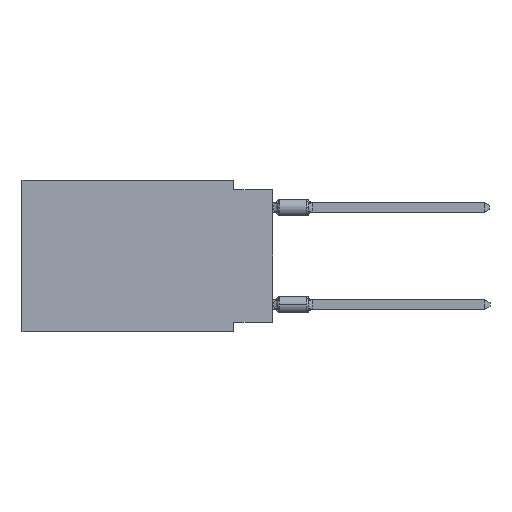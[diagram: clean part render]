
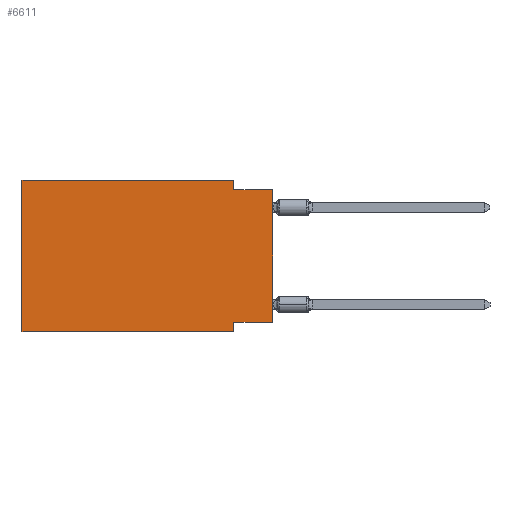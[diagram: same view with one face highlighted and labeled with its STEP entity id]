
A CAD part, left-side view. The second image highlights one B-rep face of the part: STEP entity #6611.
In plain terms, the highlighted planar face has unit normal (-1, 0, 0).
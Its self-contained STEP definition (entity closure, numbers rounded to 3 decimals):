
#212 = FACE_OUTER_BOUND ( 'NONE', #12489, .T. ) ;
#368 = LINE ( 'NONE', #21685, #13185 ) ;
#788 = VECTOR ( 'NONE', #5317, 1000. ) ;
#1435 = ORIENTED_EDGE ( 'NONE', *, *, #8250, .F. ) ;
#1480 = CARTESIAN_POINT ( 'NONE',  ( 0., 16.383, 0. ) ) ;
#1493 = CARTESIAN_POINT ( 'NONE',  ( 0., 0., -9.271 ) ) ;
#1527 = EDGE_CURVE ( 'NONE', #22306, #7343, #13561, .T. ) ;
#1873 = ORIENTED_EDGE ( 'NONE', *, *, #10326, .T. ) ;
#1948 = CARTESIAN_POINT ( 'NONE',  ( 0., 16.383, 0. ) ) ;
#1962 = CARTESIAN_POINT ( 'NONE',  ( 0., 2.54, -9.271 ) ) ;
#2350 = CARTESIAN_POINT ( 'NONE',  ( 0., 16.383, 0. ) ) ;
#2560 = DIRECTION ( 'NONE',  ( 0., 0., -1. ) ) ;
#2696 = CARTESIAN_POINT ( 'NONE',  ( 0., 16.383, -9.906 ) ) ;
#3153 = EDGE_CURVE ( 'NONE', #20212, #21137, #6985, .T. ) ;
#3161 = ORIENTED_EDGE ( 'NONE', *, *, #3596, .F. ) ;
#3207 = LINE ( 'NONE', #1480, #19437 ) ;
#3569 = VECTOR ( 'NONE', #8498, 1000. ) ;
#3596 = EDGE_CURVE ( 'NONE', #20198, #20212, #368, .T. ) ;
#3820 = EDGE_CURVE ( 'NONE', #22144, #9013, #8529, .T. ) ;
#4472 = AXIS2_PLACEMENT_3D ( 'NONE', #1948, #8731, #8949 ) ;
#5317 = DIRECTION ( 'NONE',  ( 0., 0., 1. ) ) ;
#6611 = ADVANCED_FACE ( 'NONE', ( #212 ), #10436, .F. ) ;
#6985 = LINE ( 'NONE', #20714, #8744 ) ;
#7090 = DIRECTION ( 'NONE',  ( 0., -1., 0. ) ) ;
#7343 = VERTEX_POINT ( 'NONE', #22414 ) ;
#8193 = DIRECTION ( 'NONE',  ( 0., -1., 0. ) ) ;
#8219 = ORIENTED_EDGE ( 'NONE', *, *, #3820, .F. ) ;
#8250 = EDGE_CURVE ( 'NONE', #9013, #20198, #3207, .T. ) ;
#8498 = DIRECTION ( 'NONE',  ( 0., 1., 0. ) ) ;
#8529 = LINE ( 'NONE', #10350, #10602 ) ;
#8692 = VECTOR ( 'NONE', #8193, 1000. ) ;
#8714 = ORIENTED_EDGE ( 'NONE', *, *, #3153, .F. ) ;
#8731 = DIRECTION ( 'NONE',  ( 1., 0., 0. ) ) ;
#8744 = VECTOR ( 'NONE', #7090, 1000. ) ;
#8872 = CARTESIAN_POINT ( 'NONE',  ( 0., 0., 0. ) ) ;
#8949 = DIRECTION ( 'NONE',  ( 0., 0., -1. ) ) ;
#8987 = ORIENTED_EDGE ( 'NONE', *, *, #1527, .F. ) ;
#9013 = VERTEX_POINT ( 'NONE', #2350 ) ;
#9773 = CARTESIAN_POINT ( 'NONE',  ( 0., 16.383, -9.906 ) ) ;
#10067 = CARTESIAN_POINT ( 'NONE',  ( 0., 2.54, -9.906 ) ) ;
#10326 = EDGE_CURVE ( 'NONE', #17331, #21137, #19489, .T. ) ;
#10350 = CARTESIAN_POINT ( 'NONE',  ( 0., 16.383, 0. ) ) ;
#10436 = PLANE ( 'NONE',  #4472 ) ;
#10602 = VECTOR ( 'NONE', #15788, 1000. ) ;
#12489 = EDGE_LOOP ( 'NONE', ( #1873, #8714, #3161, #1435, #8219, #15267, #8987, #15769 ) ) ;
#13185 = VECTOR ( 'NONE', #2560, 1000. ) ;
#13561 = LINE ( 'NONE', #10067, #17154 ) ;
#14243 = CARTESIAN_POINT ( 'NONE',  ( 0., 0., -0.635 ) ) ;
#15267 = ORIENTED_EDGE ( 'NONE', *, *, #15818, .T. ) ;
#15454 = CARTESIAN_POINT ( 'NONE',  ( 0., 2.54, -0.635 ) ) ;
#15508 = DIRECTION ( 'NONE',  ( 0., 0., -1. ) ) ;
#15769 = ORIENTED_EDGE ( 'NONE', *, *, #19521, .F. ) ;
#15788 = DIRECTION ( 'NONE',  ( 0., 0., 1. ) ) ;
#15818 = EDGE_CURVE ( 'NONE', #22144, #7343, #16981, .T. ) ;
#16981 = LINE ( 'NONE', #2696, #8692 ) ;
#17069 = CARTESIAN_POINT ( 'NONE',  ( 0., 0., -9.271 ) ) ;
#17154 = VECTOR ( 'NONE', #15508, 1000. ) ;
#17207 = CARTESIAN_POINT ( 'NONE',  ( 0., 2.54, 0. ) ) ;
#17290 = LINE ( 'NONE', #1493, #3569 ) ;
#17331 = VERTEX_POINT ( 'NONE', #17069 ) ;
#19437 = VECTOR ( 'NONE', #20709, 1000. ) ;
#19489 = LINE ( 'NONE', #8872, #788 ) ;
#19521 = EDGE_CURVE ( 'NONE', #17331, #22306, #17290, .T. ) ;
#20198 = VERTEX_POINT ( 'NONE', #17207 ) ;
#20212 = VERTEX_POINT ( 'NONE', #15454 ) ;
#20709 = DIRECTION ( 'NONE',  ( 0., -1., 0. ) ) ;
#20714 = CARTESIAN_POINT ( 'NONE',  ( 0., 0., -0.635 ) ) ;
#21137 = VERTEX_POINT ( 'NONE', #14243 ) ;
#21685 = CARTESIAN_POINT ( 'NONE',  ( 0., 2.54, 0. ) ) ;
#22144 = VERTEX_POINT ( 'NONE', #9773 ) ;
#22306 = VERTEX_POINT ( 'NONE', #1962 ) ;
#22414 = CARTESIAN_POINT ( 'NONE',  ( 0., 2.54, -9.906 ) ) ;
